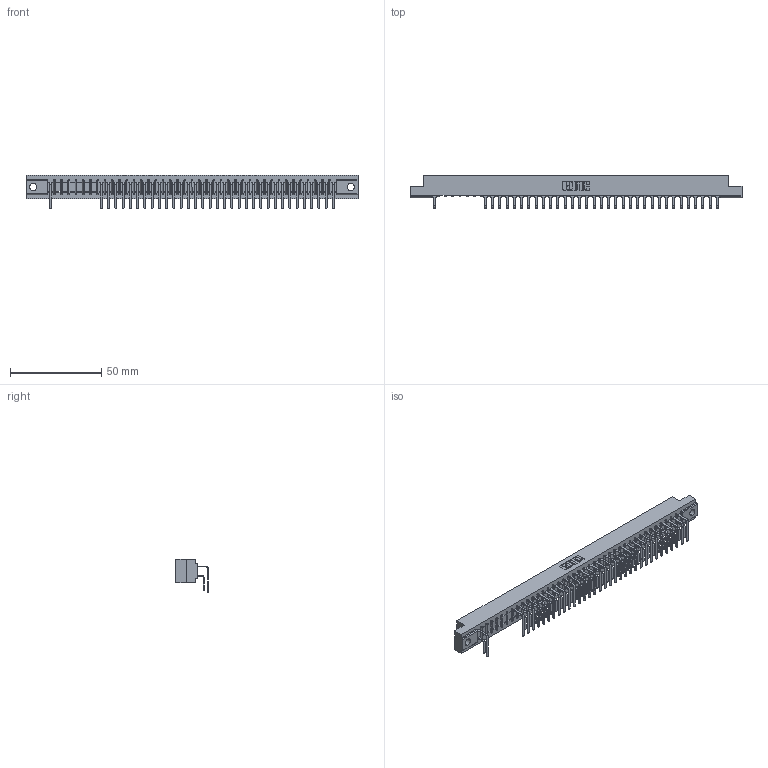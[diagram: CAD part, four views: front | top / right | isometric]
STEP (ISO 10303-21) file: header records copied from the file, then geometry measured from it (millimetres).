
FILE_DESCRIPTION (( 'STEP AP203' ), '1' );
FILE_NAME ('307-040-559-104.STEP', '2018-08-05T14:00:04', ( '' ), ( '' ), 'SwSTEP 2.0', 'SolidWorks 2016', '' );
FILE_SCHEMA (( 'CONFIG_CONTROL_DESIGN' ));
Length unit declared in the file: inch
Products named in the file (4): 307-290-001_559 - 2 (Single); 307-040-559-104; 307 Part_.156 Dia Mounting Holes; 307-290-001_558 559 - 1 (Single)
Assembly tree (68 placements, depth 2):
  307-040-559-104
    307 Part_.156 Dia Mounting Holes
    307-290-001_558 559 - 1 (Single)  x33
    307-290-001_559 - 2 (Single)  x34
Bounding box: 181.51 x 17.69 x 18.07 mm (x, y, z)
Volume: 19311.5 mm3; surface area: 24057.8 mm2
Topology: 68 solids, 68 shells, 3653 faces, 10289 edges, 6658 vertices
Faces by surface type: plane 2373, cylinder 1198, sphere 82
Entity records: 37267 total; most frequent: CARTESIAN_POINT 6159, ORIENTED_EDGE 6114, DIRECTION 6011, EDGE_CURVE 3057, VECTOR 2351, LINE 2351, VERTEX_POINT 1978, AXIS2_PLACEMENT_3D 1830
